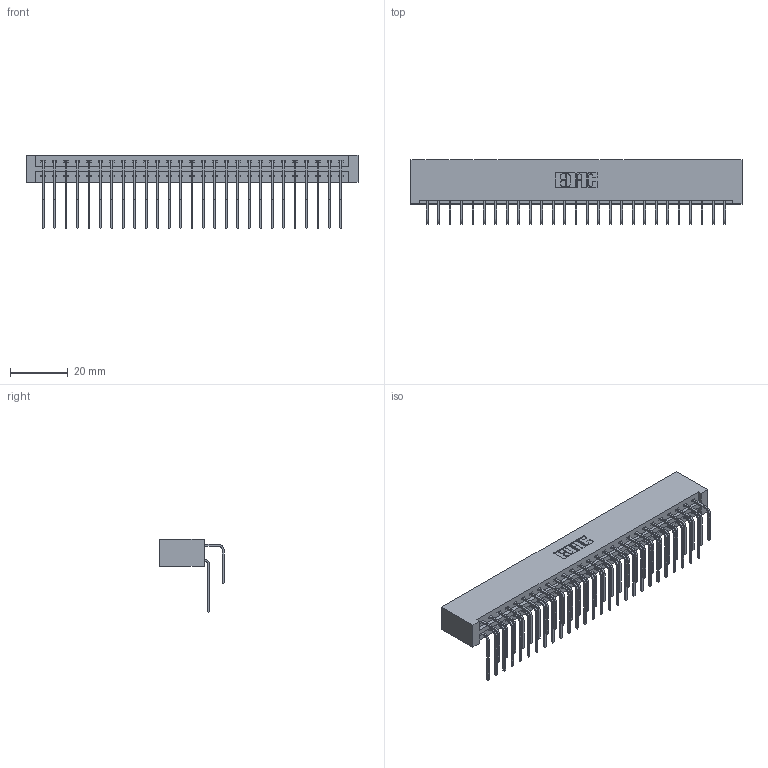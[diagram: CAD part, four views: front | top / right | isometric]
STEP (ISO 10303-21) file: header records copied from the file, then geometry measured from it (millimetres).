
FILE_DESCRIPTION (( 'STEP AP203' ), '1' );
FILE_NAME ('387-054-558-201.STEP', '2019-10-19T05:41:23', ( '' ), ( '' ), 'SwSTEP 2.0', 'SolidWorks 2016', '' );
FILE_SCHEMA (( 'CONFIG_CONTROL_DESIGN' ));
Length unit declared in the file: inch
Products named in the file (4): 345-292-001_558 Tail - 2; 387-054-558-201; 345-292-001_558 559 Tail - 1; 337 Part_No Mounting Lugs
Assembly tree (55 placements, depth 2):
  387-054-558-201
    337 Part_No Mounting Lugs
    345-292-001_558 559 Tail - 1  x27
    345-292-001_558 Tail - 2  x27
Bounding box: 114.86 x 22.17 x 25.53 mm (x, y, z)
Volume: 12977.3 mm3; surface area: 16145.4 mm2
Topology: 55 solids, 55 shells, 3130 faces, 9305 edges, 6130 vertices
Faces by surface type: plane 2226, cylinder 904
Entity records: 24381 total; most frequent: CARTESIAN_POINT 4165, ORIENTED_EDGE 4050, DIRECTION 3545, EDGE_CURVE 2025, LINE 1865, VECTOR 1865, VERTEX_POINT 1346, AXIS2_PLACEMENT_3D 840
